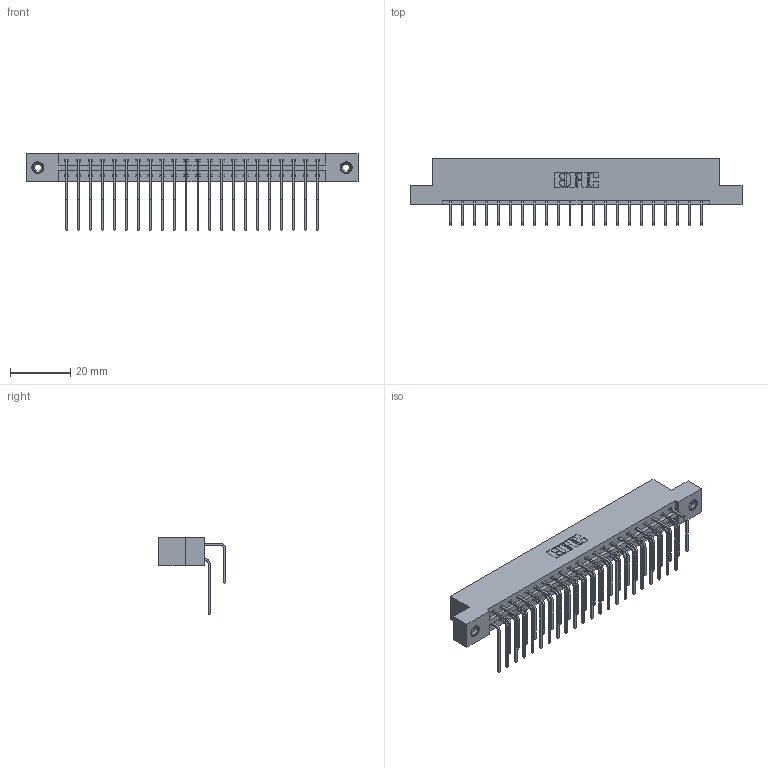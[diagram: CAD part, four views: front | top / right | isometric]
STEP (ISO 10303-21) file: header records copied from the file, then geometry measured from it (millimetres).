
FILE_DESCRIPTION (( 'STEP AP203' ), '1' );
FILE_NAME ('387-044-558-208.STEP', '2019-10-18T06:27:42', ( '' ), ( '' ), 'SwSTEP 2.0', 'SolidWorks 2016', '' );
FILE_SCHEMA (( 'CONFIG_CONTROL_DESIGN' ));
Length unit declared in the file: inch
Products named in the file (5): 387-044-558-208; 337 Part_Flush Mounting Lugs - 0.156 Dia-TI; 345-292-001_558 559 Tail - 1; 345-250-001_345-250-003-102; 345-292-001_558 Tail - 2
Assembly tree (47 placements, depth 2):
  387-044-558-208
    337 Part_Flush Mounting Lugs - 0.156 Dia-TI
    345-292-001_558 559 Tail - 1  x22
    345-292-001_558 Tail - 2  x22
    345-250-001_345-250-003-102  x2
Bounding box: 110.19 x 22.17 x 25.53 mm (x, y, z)
Volume: 11593.3 mm3; surface area: 14210.4 mm2
Topology: 47 solids, 47 shells, 2638 faces, 7795 edges, 5130 vertices
Faces by surface type: plane 1862, cylinder 760, cone 12, torus 4
Entity records: 22614 total; most frequent: CARTESIAN_POINT 3852, ORIENTED_EDGE 3730, DIRECTION 3327, EDGE_CURVE 1865, VECTOR 1677, LINE 1677, VERTEX_POINT 1236, AXIS2_PLACEMENT_3D 825
